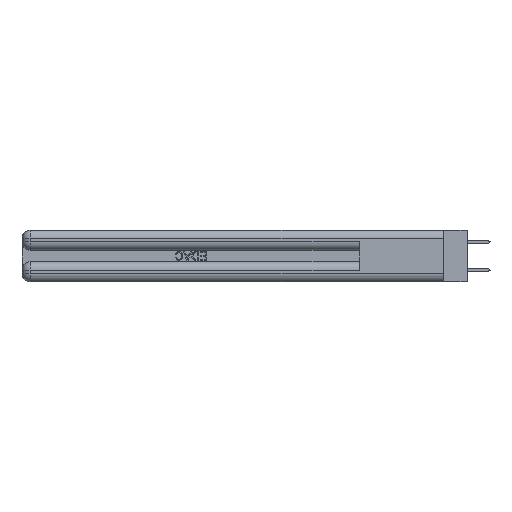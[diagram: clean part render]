
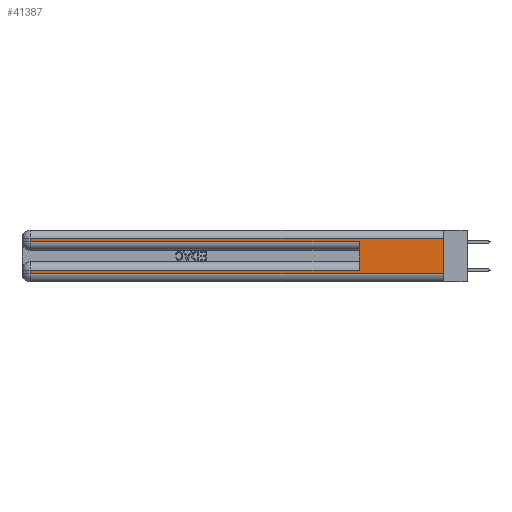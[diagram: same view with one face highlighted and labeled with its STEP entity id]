
A CAD part, left-side view. The second image highlights one B-rep face of the part: STEP entity #41387.
In plain terms, the highlighted planar face has unit normal (-1, 0, 0).
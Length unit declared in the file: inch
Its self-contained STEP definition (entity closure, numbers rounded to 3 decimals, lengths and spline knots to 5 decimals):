
#677 = EDGE_CURVE ( 'NONE', #1522, #33541, #23591, .T. ) ;
#783 = CARTESIAN_POINT ( 'NONE',  ( 0., 0.6, 0.085 ) ) ;
#1522 = VERTEX_POINT ( 'NONE', #35522 ) ;
#1942 = LINE ( 'NONE', #5857, #46678 ) ;
#4068 = VECTOR ( 'NONE', #36639, 39.37008 ) ;
#4262 = ORIENTED_EDGE ( 'NONE', *, *, #26618, .F. ) ;
#4786 = DIRECTION ( 'NONE',  ( 0., 0., -1. ) ) ;
#5857 = CARTESIAN_POINT ( 'NONE',  ( 0., 0., 0.31 ) ) ;
#6078 = VECTOR ( 'NONE', #44587, 39.37008 ) ;
#6592 = VECTOR ( 'NONE', #26335, 39.37008 ) ;
#6665 = AXIS2_PLACEMENT_3D ( 'NONE', #40242, #9752, #25242 ) ;
#7068 = ORIENTED_EDGE ( 'NONE', *, *, #677, .T. ) ;
#8351 = CARTESIAN_POINT ( 'NONE',  ( 0., 0., 0.285 ) ) ;
#8657 = VECTOR ( 'NONE', #43282, 39.37008 ) ;
#9752 = DIRECTION ( 'NONE',  ( 1., 0., 0. ) ) ;
#10240 = CARTESIAN_POINT ( 'NONE',  ( 0., 0., 0.085 ) ) ;
#10533 = CARTESIAN_POINT ( 'NONE',  ( 0., 2.94, 0.31 ) ) ;
#12473 = CARTESIAN_POINT ( 'NONE',  ( 0., 0., 0.06 ) ) ;
#14629 = EDGE_CURVE ( 'NONE', #33541, #18549, #28295, .T. ) ;
#14643 = VECTOR ( 'NONE', #15546, 39.37008 ) ;
#15546 = DIRECTION ( 'NONE',  ( 0., 0., -1. ) ) ;
#15748 = VERTEX_POINT ( 'NONE', #31300 ) ;
#16706 = ORIENTED_EDGE ( 'NONE', *, *, #14629, .T. ) ;
#18549 = VERTEX_POINT ( 'NONE', #12473 ) ;
#19702 = CARTESIAN_POINT ( 'NONE',  ( 0., 2.94, 0.37 ) ) ;
#20465 = EDGE_LOOP ( 'NONE', ( #39962, #48517, #28672, #23888, #4262, #48924, #7068, #16706 ) ) ;
#21030 = DIRECTION ( 'NONE',  ( 0., 1., 0. ) ) ;
#21858 = VERTEX_POINT ( 'NONE', #21960 ) ;
#21960 = CARTESIAN_POINT ( 'NONE',  ( 0., 2.94, 0.285 ) ) ;
#23591 = LINE ( 'NONE', #19702, #14643 ) ;
#23866 = VECTOR ( 'NONE', #4786, 39.37008 ) ;
#23888 = ORIENTED_EDGE ( 'NONE', *, *, #36537, .T. ) ;
#24366 = LINE ( 'NONE', #47394, #4068 ) ;
#24887 = EDGE_CURVE ( 'NONE', #37236, #1522, #28727, .T. ) ;
#25242 = DIRECTION ( 'NONE',  ( 0., 0., -1. ) ) ;
#25329 = CARTESIAN_POINT ( 'NONE',  ( 0., 2.94, 0.06 ) ) ;
#25399 = PLANE ( 'NONE',  #6665 ) ;
#25869 = EDGE_CURVE ( 'NONE', #36446, #21858, #26842, .T. ) ;
#26335 = DIRECTION ( 'NONE',  ( 0., 0., -1. ) ) ;
#26618 = EDGE_CURVE ( 'NONE', #37236, #30432, #24366, .T. ) ;
#26842 = LINE ( 'NONE', #31137, #23866 ) ;
#26977 = EDGE_CURVE ( 'NONE', #15748, #36446, #1942, .T. ) ;
#26997 = FACE_OUTER_BOUND ( 'NONE', #20465, .T. ) ;
#27525 = DIRECTION ( 'NONE',  ( 0., -1., 0. ) ) ;
#27923 = CARTESIAN_POINT ( 'NONE',  ( 0., 0., 0.06 ) ) ;
#28295 = LINE ( 'NONE', #27923, #8657 ) ;
#28672 = ORIENTED_EDGE ( 'NONE', *, *, #25869, .T. ) ;
#28727 = LINE ( 'NONE', #10240, #6078 ) ;
#29239 = LINE ( 'NONE', #29648, #6592 ) ;
#29648 = CARTESIAN_POINT ( 'NONE',  ( 0., 0., 0.37 ) ) ;
#30432 = VERTEX_POINT ( 'NONE', #35113 ) ;
#31137 = CARTESIAN_POINT ( 'NONE',  ( 0., 2.94, 0.37 ) ) ;
#31300 = CARTESIAN_POINT ( 'NONE',  ( 0., 0., 0.31 ) ) ;
#33541 = VERTEX_POINT ( 'NONE', #25329 ) ;
#35113 = CARTESIAN_POINT ( 'NONE',  ( 0., 0.6, 0.285 ) ) ;
#35522 = CARTESIAN_POINT ( 'NONE',  ( 0., 2.94, 0.085 ) ) ;
#36446 = VERTEX_POINT ( 'NONE', #10533 ) ;
#36537 = EDGE_CURVE ( 'NONE', #21858, #30432, #46871, .T. ) ;
#36639 = DIRECTION ( 'NONE',  ( 0., 0., 1. ) ) ;
#37236 = VERTEX_POINT ( 'NONE', #783 ) ;
#39962 = ORIENTED_EDGE ( 'NONE', *, *, #47614, .F. ) ;
#40242 = CARTESIAN_POINT ( 'NONE',  ( 0., 0., 0.37 ) ) ;
#41387 = ADVANCED_FACE ( 'NONE', ( #26997 ), #25399, .F. ) ;
#43282 = DIRECTION ( 'NONE',  ( 0., -1., 0. ) ) ;
#44587 = DIRECTION ( 'NONE',  ( 0., 1., 0. ) ) ;
#45027 = VECTOR ( 'NONE', #27525, 39.37008 ) ;
#46678 = VECTOR ( 'NONE', #21030, 39.37008 ) ;
#46871 = LINE ( 'NONE', #8351, #45027 ) ;
#47394 = CARTESIAN_POINT ( 'NONE',  ( 0., 0.6, 0.145 ) ) ;
#47614 = EDGE_CURVE ( 'NONE', #15748, #18549, #29239, .T. ) ;
#48517 = ORIENTED_EDGE ( 'NONE', *, *, #26977, .T. ) ;
#48924 = ORIENTED_EDGE ( 'NONE', *, *, #24887, .T. ) ;
